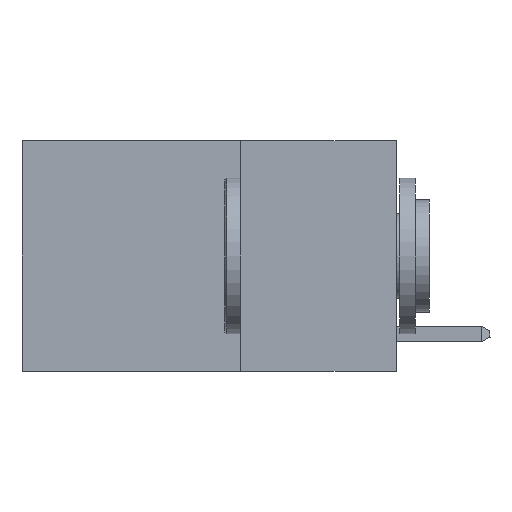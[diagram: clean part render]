
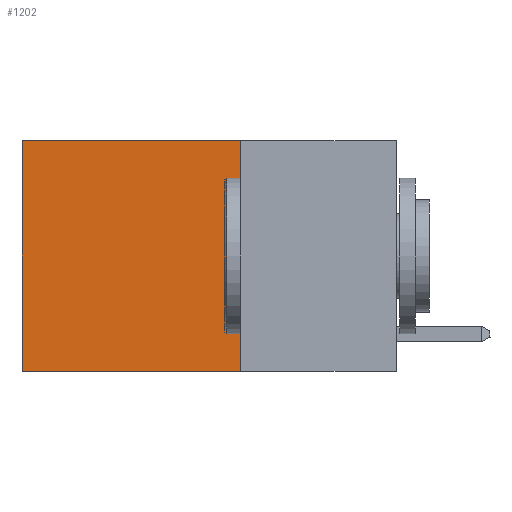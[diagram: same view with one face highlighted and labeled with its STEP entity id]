
A CAD part, left-side view. The second image highlights one B-rep face of the part: STEP entity #1202.
In plain terms, the highlighted planar face has unit normal (-1, 0, 0).
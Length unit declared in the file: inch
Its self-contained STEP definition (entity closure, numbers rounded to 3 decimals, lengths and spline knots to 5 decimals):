
#57 = EDGE_LOOP ( 'NONE', ( #188, #2856, #8798, #6576 ) ) ;
#188 = ORIENTED_EDGE ( 'NONE', *, *, #792, .T. ) ;
#313 = VECTOR ( 'NONE', #7479, 39.37008 ) ;
#345 = CARTESIAN_POINT ( 'NONE',  ( 0.2625, 0.25, 0. ) ) ;
#792 = EDGE_CURVE ( 'NONE', #2962, #5741, #1098, .T. ) ;
#1098 = LINE ( 'NONE', #3916, #7601 ) ;
#1202 = ADVANCED_FACE ( 'NONE', ( #6229 ), #9245, .F. ) ;
#1209 = EDGE_CURVE ( 'NONE', #7932, #2962, #8482, .T. ) ;
#2197 = VERTEX_POINT ( 'NONE', #2750 ) ;
#2750 = CARTESIAN_POINT ( 'NONE',  ( 0.2625, 0.25, -0.37 ) ) ;
#2856 = ORIENTED_EDGE ( 'NONE', *, *, #8993, .F. ) ;
#2962 = VERTEX_POINT ( 'NONE', #9261 ) ;
#3380 = AXIS2_PLACEMENT_3D ( 'NONE', #345, #4886, #4101 ) ;
#3538 = CARTESIAN_POINT ( 'NONE',  ( 0.2625, 0.6, -0.37 ) ) ;
#3867 = EDGE_CURVE ( 'NONE', #7932, #2197, #4429, .T. ) ;
#3916 = CARTESIAN_POINT ( 'NONE',  ( 0.2625, 0.6, 0. ) ) ;
#4051 = DIRECTION ( 'NONE',  ( 0., 0., -1. ) ) ;
#4101 = DIRECTION ( 'NONE',  ( 0., 0., -1. ) ) ;
#4429 = LINE ( 'NONE', #5280, #313 ) ;
#4600 = DIRECTION ( 'NONE',  ( 0., 1., 0. ) ) ;
#4794 = DIRECTION ( 'NONE',  ( 0., 1., 0. ) ) ;
#4886 = DIRECTION ( 'NONE',  ( 1., 0., 0. ) ) ;
#4900 = VECTOR ( 'NONE', #4600, 39.37008 ) ;
#5280 = CARTESIAN_POINT ( 'NONE',  ( 0.2625, 0.25, 0. ) ) ;
#5741 = VERTEX_POINT ( 'NONE', #3538 ) ;
#5950 = LINE ( 'NONE', #6054, #4900 ) ;
#6054 = CARTESIAN_POINT ( 'NONE',  ( 0.2625, 0.25, -0.37 ) ) ;
#6153 = CARTESIAN_POINT ( 'NONE',  ( 0.2625, 0.25, 0. ) ) ;
#6229 = FACE_OUTER_BOUND ( 'NONE', #57, .T. ) ;
#6318 = CARTESIAN_POINT ( 'NONE',  ( 0.2625, 0.25, 0. ) ) ;
#6576 = ORIENTED_EDGE ( 'NONE', *, *, #1209, .T. ) ;
#7479 = DIRECTION ( 'NONE',  ( 0., 0., -1. ) ) ;
#7601 = VECTOR ( 'NONE', #4051, 39.37008 ) ;
#7932 = VERTEX_POINT ( 'NONE', #6153 ) ;
#8263 = VECTOR ( 'NONE', #4794, 39.37008 ) ;
#8482 = LINE ( 'NONE', #6318, #8263 ) ;
#8798 = ORIENTED_EDGE ( 'NONE', *, *, #3867, .F. ) ;
#8993 = EDGE_CURVE ( 'NONE', #2197, #5741, #5950, .T. ) ;
#9245 = PLANE ( 'NONE',  #3380 ) ;
#9261 = CARTESIAN_POINT ( 'NONE',  ( 0.2625, 0.6, 0. ) ) ;
